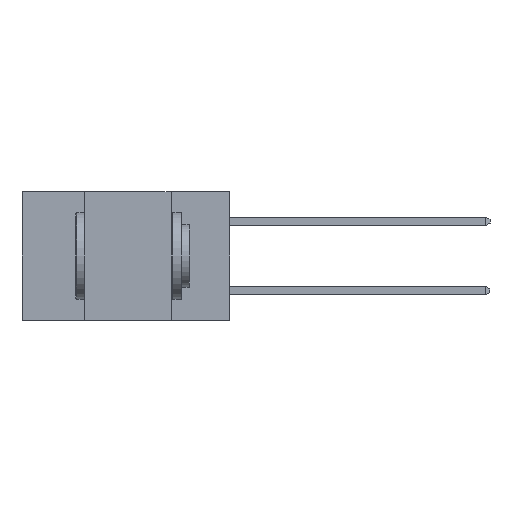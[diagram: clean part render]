
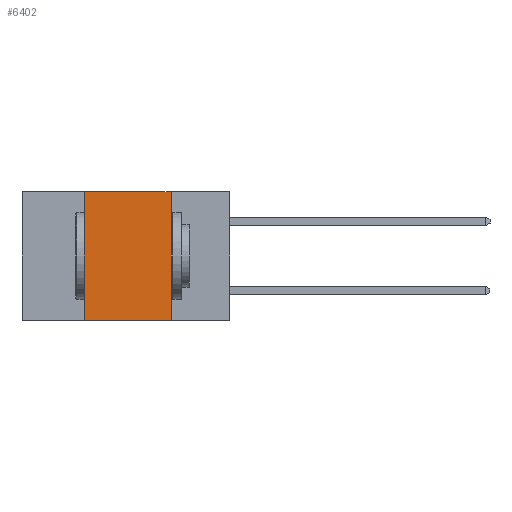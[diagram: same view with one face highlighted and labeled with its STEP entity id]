
A CAD part, left-side view. The second image highlights one B-rep face of the part: STEP entity #6402.
In plain terms, the highlighted planar face has unit normal (-1, 0, 0).
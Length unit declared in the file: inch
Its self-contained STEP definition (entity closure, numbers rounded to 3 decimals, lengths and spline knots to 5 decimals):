
#24 = EDGE_LOOP ( 'NONE', ( #414, #1452, #18340, #7273 ) ) ;
#414 = ORIENTED_EDGE ( 'NONE', *, *, #16203, .F. ) ;
#972 = CARTESIAN_POINT ( 'NONE',  ( 0., 0.42, 0. ) ) ;
#1299 = LINE ( 'NONE', #18251, #5630 ) ;
#1413 = VECTOR ( 'NONE', #14196, 39.37008 ) ;
#1452 = ORIENTED_EDGE ( 'NONE', *, *, #1486, .F. ) ;
#1486 = EDGE_CURVE ( 'NONE', #4429, #10935, #1299, .T. ) ;
#1525 = CARTESIAN_POINT ( 'NONE',  ( 0., 0.17, 0. ) ) ;
#2729 = VERTEX_POINT ( 'NONE', #15999 ) ;
#2865 = EDGE_CURVE ( 'NONE', #2729, #14889, #8719, .T. ) ;
#3051 = CARTESIAN_POINT ( 'NONE',  ( 0., 0.6, 0. ) ) ;
#3193 = DIRECTION ( 'NONE',  ( 0., 0., -1. ) ) ;
#3378 = LINE ( 'NONE', #1525, #11314 ) ;
#3721 = DIRECTION ( 'NONE',  ( 1., 0., 0. ) ) ;
#4429 = VERTEX_POINT ( 'NONE', #972 ) ;
#4854 = CARTESIAN_POINT ( 'NONE',  ( 0., 0.17, 0. ) ) ;
#5630 = VECTOR ( 'NONE', #14746, 39.37008 ) ;
#6314 = CARTESIAN_POINT ( 'NONE',  ( 0., 0.17, -0.37 ) ) ;
#6402 = ADVANCED_FACE ( 'NONE', ( #13069 ), #9332, .F. ) ;
#7273 = ORIENTED_EDGE ( 'NONE', *, *, #2865, .T. ) ;
#8719 = LINE ( 'NONE', #13477, #16676 ) ;
#9332 = PLANE ( 'NONE',  #10912 ) ;
#9911 = LINE ( 'NONE', #12569, #1413 ) ;
#10912 = AXIS2_PLACEMENT_3D ( 'NONE', #3051, #3721, #13276 ) ;
#10935 = VERTEX_POINT ( 'NONE', #4854 ) ;
#11314 = VECTOR ( 'NONE', #3193, 39.37008 ) ;
#12569 = CARTESIAN_POINT ( 'NONE',  ( 0., 0.42, 0. ) ) ;
#13069 = FACE_OUTER_BOUND ( 'NONE', #24, .T. ) ;
#13276 = DIRECTION ( 'NONE',  ( 0., 0., -1. ) ) ;
#13477 = CARTESIAN_POINT ( 'NONE',  ( 0., 0.6, -0.37 ) ) ;
#14196 = DIRECTION ( 'NONE',  ( 0., 0., 1. ) ) ;
#14746 = DIRECTION ( 'NONE',  ( 0., -1., 0. ) ) ;
#14889 = VERTEX_POINT ( 'NONE', #6314 ) ;
#15999 = CARTESIAN_POINT ( 'NONE',  ( 0., 0.42, -0.37 ) ) ;
#16203 = EDGE_CURVE ( 'NONE', #10935, #14889, #3378, .T. ) ;
#16454 = DIRECTION ( 'NONE',  ( 0., -1., 0. ) ) ;
#16676 = VECTOR ( 'NONE', #16454, 39.37008 ) ;
#18251 = CARTESIAN_POINT ( 'NONE',  ( 0., 0.6, 0. ) ) ;
#18340 = ORIENTED_EDGE ( 'NONE', *, *, #20086, .F. ) ;
#20086 = EDGE_CURVE ( 'NONE', #2729, #4429, #9911, .T. ) ;
